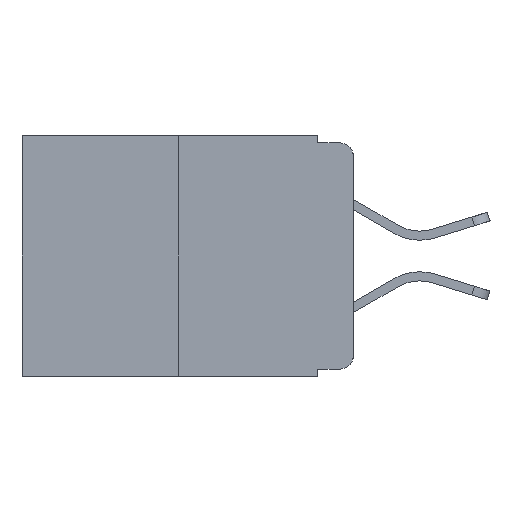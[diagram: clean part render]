
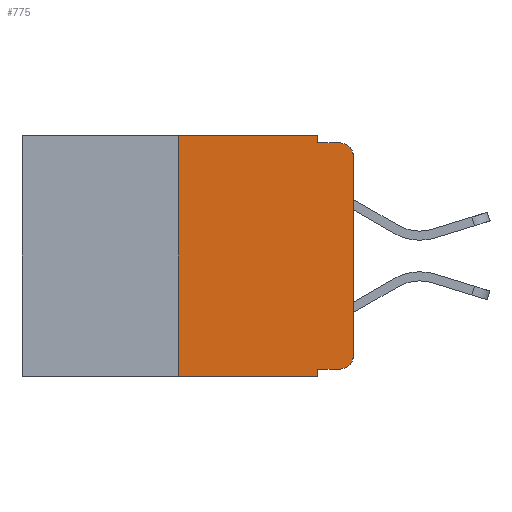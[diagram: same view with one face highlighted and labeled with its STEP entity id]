
A CAD part, left-side view. The second image highlights one B-rep face of the part: STEP entity #775.
In plain terms, the highlighted planar face has unit normal (-1, 0, 0).
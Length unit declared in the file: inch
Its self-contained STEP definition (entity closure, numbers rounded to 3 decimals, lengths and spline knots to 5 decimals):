
#344 = VECTOR ( 'NONE', #12935, 39.37008 ) ;
#474 = VERTEX_POINT ( 'NONE', #5316 ) ;
#775 = ADVANCED_FACE ( 'NONE', ( #14812 ), #12518, .F. ) ;
#906 = DIRECTION ( 'NONE',  ( 0., -1., 0. ) ) ;
#1118 = EDGE_CURVE ( 'NONE', #8353, #13649, #7659, .T. ) ;
#1229 = VERTEX_POINT ( 'NONE', #3002 ) ;
#1395 = VERTEX_POINT ( 'NONE', #7193 ) ;
#2063 = LINE ( 'NONE', #2803, #17501 ) ;
#2203 = VERTEX_POINT ( 'NONE', #14372 ) ;
#2204 = EDGE_CURVE ( 'NONE', #8090, #1395, #2063, .T. ) ;
#2373 = CARTESIAN_POINT ( 'NONE',  ( 0., 0.051, 0. ) ) ;
#2507 = LINE ( 'NONE', #11026, #3481 ) ;
#2664 = CIRCLE ( 'NONE', #14080, 0.02 ) ;
#2803 = CARTESIAN_POINT ( 'NONE',  ( 0., 0.25, 0. ) ) ;
#3002 = CARTESIAN_POINT ( 'NONE',  ( 0., 0.02, -0.333 ) ) ;
#3255 = EDGE_CURVE ( 'NONE', #8510, #4122, #4224, .T. ) ;
#3481 = VECTOR ( 'NONE', #12503, 39.37008 ) ;
#4122 = VERTEX_POINT ( 'NONE', #16395 ) ;
#4224 = LINE ( 'NONE', #6379, #12240 ) ;
#4299 = EDGE_CURVE ( 'NONE', #4122, #474, #4428, .T. ) ;
#4428 = LINE ( 'NONE', #13492, #11966 ) ;
#4655 = AXIS2_PLACEMENT_3D ( 'NONE', #11797, #10348, #10493 ) ;
#4689 = DIRECTION ( 'NONE',  ( -1., 0., 0. ) ) ;
#5308 = EDGE_CURVE ( 'NONE', #6049, #474, #2664, .T. ) ;
#5316 = CARTESIAN_POINT ( 'NONE',  ( 0., 0.02, -0.01 ) ) ;
#5426 = ORIENTED_EDGE ( 'NONE', *, *, #18521, .T. ) ;
#6049 = VERTEX_POINT ( 'NONE', #11182 ) ;
#6163 = ORIENTED_EDGE ( 'NONE', *, *, #1118, .F. ) ;
#6362 = ORIENTED_EDGE ( 'NONE', *, *, #13952, .T. ) ;
#6379 = CARTESIAN_POINT ( 'NONE',  ( 0., 0.051, 0. ) ) ;
#7193 = CARTESIAN_POINT ( 'NONE',  ( 0., 0.25, 0. ) ) ;
#7235 = DIRECTION ( 'NONE',  ( -1., 0., 0. ) ) ;
#7377 = EDGE_CURVE ( 'NONE', #2203, #6049, #16477, .T. ) ;
#7659 = LINE ( 'NONE', #2373, #19278 ) ;
#7960 = ORIENTED_EDGE ( 'NONE', *, *, #2204, .F. ) ;
#8090 = VERTEX_POINT ( 'NONE', #16308 ) ;
#8353 = VERTEX_POINT ( 'NONE', #18248 ) ;
#8510 = VERTEX_POINT ( 'NONE', #17155 ) ;
#8653 = ORIENTED_EDGE ( 'NONE', *, *, #17595, .T. ) ;
#9980 = ORIENTED_EDGE ( 'NONE', *, *, #4299, .F. ) ;
#10163 = VECTOR ( 'NONE', #906, 39.37008 ) ;
#10348 = DIRECTION ( 'NONE',  ( 1., 0., 0. ) ) ;
#10493 = DIRECTION ( 'NONE',  ( 0., 0., -1. ) ) ;
#11026 = CARTESIAN_POINT ( 'NONE',  ( 0., 0.473, 0. ) ) ;
#11182 = CARTESIAN_POINT ( 'NONE',  ( 0., 0., -0.03 ) ) ;
#11262 = EDGE_CURVE ( 'NONE', #1395, #8510, #2507, .T. ) ;
#11465 = VECTOR ( 'NONE', #12964, 39.37008 ) ;
#11488 = CARTESIAN_POINT ( 'NONE',  ( 0., 0.473, -0.343 ) ) ;
#11797 = CARTESIAN_POINT ( 'NONE',  ( 0., 0.473, 0. ) ) ;
#11966 = VECTOR ( 'NONE', #13629, 39.37008 ) ;
#12048 = CIRCLE ( 'NONE', #15327, 0.02 ) ;
#12240 = VECTOR ( 'NONE', #13791, 39.37008 ) ;
#12503 = DIRECTION ( 'NONE',  ( 0., -1., 0. ) ) ;
#12518 = PLANE ( 'NONE',  #4655 ) ;
#12935 = DIRECTION ( 'NONE',  ( 0., 0., 1. ) ) ;
#12964 = DIRECTION ( 'NONE',  ( 0., -1., 0. ) ) ;
#13492 = CARTESIAN_POINT ( 'NONE',  ( 0., 0.051, -0.01 ) ) ;
#13629 = DIRECTION ( 'NONE',  ( 0., -1., 0. ) ) ;
#13649 = VERTEX_POINT ( 'NONE', #15094 ) ;
#13652 = CARTESIAN_POINT ( 'NONE',  ( 0., 0.02, -0.313 ) ) ;
#13791 = DIRECTION ( 'NONE',  ( 0., 0., -1. ) ) ;
#13952 = EDGE_CURVE ( 'NONE', #8090, #13649, #15367, .T. ) ;
#14012 = DIRECTION ( 'NONE',  ( 0., 0., 1. ) ) ;
#14080 = AXIS2_PLACEMENT_3D ( 'NONE', #17512, #7235, #16098 ) ;
#14372 = CARTESIAN_POINT ( 'NONE',  ( 0., 0., -0.313 ) ) ;
#14393 = CARTESIAN_POINT ( 'NONE',  ( 0., 0., 0. ) ) ;
#14511 = LINE ( 'NONE', #18794, #10163 ) ;
#14812 = FACE_OUTER_BOUND ( 'NONE', #14930, .T. ) ;
#14841 = ORIENTED_EDGE ( 'NONE', *, *, #5308, .T. ) ;
#14930 = EDGE_LOOP ( 'NONE', ( #15081, #14841, #9980, #18570, #17754, #7960, #6362, #6163, #5426, #8653 ) ) ;
#15081 = ORIENTED_EDGE ( 'NONE', *, *, #7377, .T. ) ;
#15094 = CARTESIAN_POINT ( 'NONE',  ( 0., 0.051, -0.343 ) ) ;
#15129 = DIRECTION ( 'NONE',  ( 0., 0., -1. ) ) ;
#15327 = AXIS2_PLACEMENT_3D ( 'NONE', #13652, #4689, #15129 ) ;
#15367 = LINE ( 'NONE', #11488, #11465 ) ;
#16098 = DIRECTION ( 'NONE',  ( 0., 0., -1. ) ) ;
#16192 = DIRECTION ( 'NONE',  ( 0., 0., -1. ) ) ;
#16308 = CARTESIAN_POINT ( 'NONE',  ( 0., 0.25, -0.343 ) ) ;
#16395 = CARTESIAN_POINT ( 'NONE',  ( 0., 0.051, -0.01 ) ) ;
#16477 = LINE ( 'NONE', #14393, #344 ) ;
#17155 = CARTESIAN_POINT ( 'NONE',  ( 0., 0.051, 0. ) ) ;
#17501 = VECTOR ( 'NONE', #14012, 39.37008 ) ;
#17512 = CARTESIAN_POINT ( 'NONE',  ( 0., 0.02, -0.03 ) ) ;
#17595 = EDGE_CURVE ( 'NONE', #1229, #2203, #12048, .T. ) ;
#17754 = ORIENTED_EDGE ( 'NONE', *, *, #11262, .F. ) ;
#18248 = CARTESIAN_POINT ( 'NONE',  ( 0., 0.051, -0.333 ) ) ;
#18521 = EDGE_CURVE ( 'NONE', #8353, #1229, #14511, .T. ) ;
#18570 = ORIENTED_EDGE ( 'NONE', *, *, #3255, .F. ) ;
#18794 = CARTESIAN_POINT ( 'NONE',  ( 0., 0.051, -0.333 ) ) ;
#19278 = VECTOR ( 'NONE', #16192, 39.37008 ) ;
